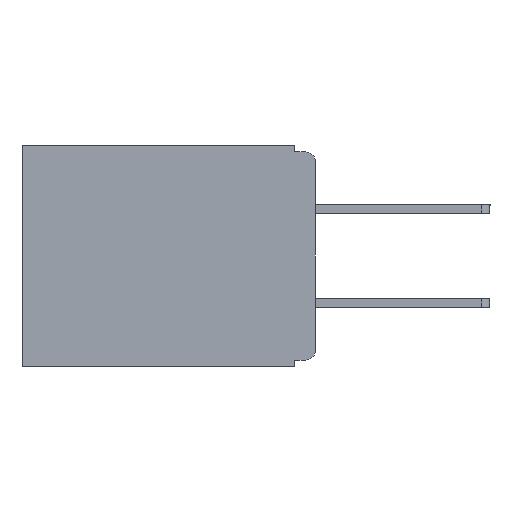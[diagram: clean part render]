
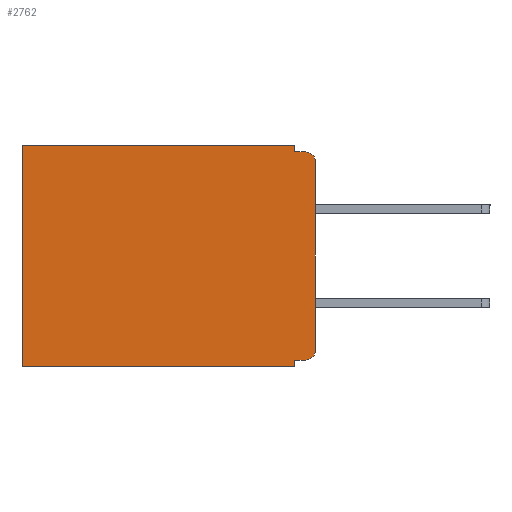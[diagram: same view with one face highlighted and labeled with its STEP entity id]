
A CAD part, left-side view. The second image highlights one B-rep face of the part: STEP entity #2762.
In plain terms, the highlighted planar face has unit normal (-1, 0, 0).
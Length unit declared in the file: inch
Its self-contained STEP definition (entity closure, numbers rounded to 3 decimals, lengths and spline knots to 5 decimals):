
#59 = CARTESIAN_POINT ( 'NONE',  ( 0.3, 0., -0.33 ) ) ;
#612 = CARTESIAN_POINT ( 'NONE',  ( 0.3, 0.015, -0.305 ) ) ;
#1297 = FACE_OUTER_BOUND ( 'NONE', #2068, .T. ) ;
#1448 = ORIENTED_EDGE ( 'NONE', *, *, #30061, .T. ) ;
#1868 = EDGE_CURVE ( 'NONE', #29486, #16507, #29975, .T. ) ;
#2068 = EDGE_LOOP ( 'NONE', ( #18898, #1448, #10422, #10959, #26774, #23212, #26796, #8528, #10632, #19428 ) ) ;
#2762 = ADVANCED_FACE ( 'NONE', ( #1297 ), #14230, .F. ) ;
#3107 = DIRECTION ( 'NONE',  ( 0., 0., -1. ) ) ;
#4763 = CARTESIAN_POINT ( 'NONE',  ( 0.3, 0., -0.305 ) ) ;
#4853 = EDGE_CURVE ( 'NONE', #28722, #25468, #7602, .T. ) ;
#6275 = VECTOR ( 'NONE', #17527, 39.37008 ) ;
#6367 = CARTESIAN_POINT ( 'NONE',  ( 0.3, 0., -0.32 ) ) ;
#6428 = CIRCLE ( 'NONE', #27168, 0.015 ) ;
#6595 = VERTEX_POINT ( 'NONE', #8997 ) ;
#6731 = DIRECTION ( 'NONE',  ( 0., 1., 0. ) ) ;
#6753 = CARTESIAN_POINT ( 'NONE',  ( 0.3, 0., -0.33 ) ) ;
#6764 = CARTESIAN_POINT ( 'NONE',  ( 0.3, 0.437, 0. ) ) ;
#6774 = LINE ( 'NONE', #8941, #23721 ) ;
#6775 = VECTOR ( 'NONE', #29089, 39.37008 ) ;
#6776 = LINE ( 'NONE', #6753, #12218 ) ;
#7475 = VERTEX_POINT ( 'NONE', #7831 ) ;
#7602 = LINE ( 'NONE', #6367, #13026 ) ;
#7777 = LINE ( 'NONE', #14402, #19295 ) ;
#7831 = CARTESIAN_POINT ( 'NONE',  ( 0.3, 0.031, -0.33 ) ) ;
#7839 = DIRECTION ( 'NONE',  ( 1., 0., 0. ) ) ;
#8376 = CARTESIAN_POINT ( 'NONE',  ( 0.3, 0., -0.01 ) ) ;
#8528 = ORIENTED_EDGE ( 'NONE', *, *, #25667, .F. ) ;
#8941 = CARTESIAN_POINT ( 'NONE',  ( 0.3, 0., 0. ) ) ;
#8997 = CARTESIAN_POINT ( 'NONE',  ( 0.3, 0.015, -0.01 ) ) ;
#9404 = AXIS2_PLACEMENT_3D ( 'NONE', #59, #7839, #13425 ) ;
#10422 = ORIENTED_EDGE ( 'NONE', *, *, #12628, .F. ) ;
#10632 = ORIENTED_EDGE ( 'NONE', *, *, #4853, .F. ) ;
#10792 = VERTEX_POINT ( 'NONE', #21966 ) ;
#10959 = ORIENTED_EDGE ( 'NONE', *, *, #27193, .F. ) ;
#11281 = DIRECTION ( 'NONE',  ( 0., 1., 0. ) ) ;
#11301 = VERTEX_POINT ( 'NONE', #16894 ) ;
#12197 = CIRCLE ( 'NONE', #25722, 0.015 ) ;
#12218 = VECTOR ( 'NONE', #18340, 39.37008 ) ;
#12562 = CARTESIAN_POINT ( 'NONE',  ( 0.3, 0.015, -0.025 ) ) ;
#12628 = EDGE_CURVE ( 'NONE', #19249, #6595, #17962, .T. ) ;
#12634 = CARTESIAN_POINT ( 'NONE',  ( 0.3, 0., -0.33 ) ) ;
#12815 = EDGE_CURVE ( 'NONE', #7475, #16507, #6776, .T. ) ;
#12888 = CARTESIAN_POINT ( 'NONE',  ( 0.3, 0.437, -0.33 ) ) ;
#13026 = VECTOR ( 'NONE', #6731, 39.37008 ) ;
#13425 = DIRECTION ( 'NONE',  ( 0., 0., -1. ) ) ;
#14230 = PLANE ( 'NONE',  #9404 ) ;
#14402 = CARTESIAN_POINT ( 'NONE',  ( 0.3, 0.031, 0. ) ) ;
#14833 = DIRECTION ( 'NONE',  ( 0., 0., -1. ) ) ;
#16507 = VERTEX_POINT ( 'NONE', #12888 ) ;
#16696 = DIRECTION ( 'NONE',  ( 0., 0., -1. ) ) ;
#16894 = CARTESIAN_POINT ( 'NONE',  ( 0.3, 0., -0.025 ) ) ;
#16998 = DIRECTION ( 'NONE',  ( -1., 0., 0. ) ) ;
#17232 = VECTOR ( 'NONE', #17438, 39.37008 ) ;
#17438 = DIRECTION ( 'NONE',  ( 0., -1., 0. ) ) ;
#17527 = DIRECTION ( 'NONE',  ( 0., 0., -1. ) ) ;
#17594 = CARTESIAN_POINT ( 'NONE',  ( 0.3, 0.031, -0.01 ) ) ;
#17962 = LINE ( 'NONE', #8376, #17232 ) ;
#18340 = DIRECTION ( 'NONE',  ( 0., 1., 0. ) ) ;
#18898 = ORIENTED_EDGE ( 'NONE', *, *, #20298, .F. ) ;
#19249 = VERTEX_POINT ( 'NONE', #17594 ) ;
#19295 = VECTOR ( 'NONE', #16696, 39.37008 ) ;
#19428 = ORIENTED_EDGE ( 'NONE', *, *, #25488, .T. ) ;
#19701 = CARTESIAN_POINT ( 'NONE',  ( 0.3, 0.437, -0.33 ) ) ;
#19743 = LINE ( 'NONE', #24447, #6775 ) ;
#19780 = CARTESIAN_POINT ( 'NONE',  ( 0.3, 0.015, -0.32 ) ) ;
#20298 = EDGE_CURVE ( 'NONE', #11301, #22526, #27330, .T. ) ;
#20519 = VECTOR ( 'NONE', #26351, 39.37008 ) ;
#21203 = EDGE_CURVE ( 'NONE', #10792, #29486, #6774, .T. ) ;
#21966 = CARTESIAN_POINT ( 'NONE',  ( 0.3, 0.031, 0. ) ) ;
#22526 = VERTEX_POINT ( 'NONE', #4763 ) ;
#23212 = ORIENTED_EDGE ( 'NONE', *, *, #1868, .T. ) ;
#23721 = VECTOR ( 'NONE', #11281, 39.37008 ) ;
#24447 = CARTESIAN_POINT ( 'NONE',  ( 0.3, 0.031, -0.33 ) ) ;
#25468 = VERTEX_POINT ( 'NONE', #28300 ) ;
#25488 = EDGE_CURVE ( 'NONE', #28722, #22526, #6428, .T. ) ;
#25667 = EDGE_CURVE ( 'NONE', #25468, #7475, #19743, .T. ) ;
#25722 = AXIS2_PLACEMENT_3D ( 'NONE', #12562, #28560, #14833 ) ;
#26351 = DIRECTION ( 'NONE',  ( 0., 0., -1. ) ) ;
#26774 = ORIENTED_EDGE ( 'NONE', *, *, #21203, .T. ) ;
#26796 = ORIENTED_EDGE ( 'NONE', *, *, #12815, .F. ) ;
#27168 = AXIS2_PLACEMENT_3D ( 'NONE', #612, #16998, #3107 ) ;
#27193 = EDGE_CURVE ( 'NONE', #10792, #19249, #7777, .T. ) ;
#27330 = LINE ( 'NONE', #12634, #20519 ) ;
#28300 = CARTESIAN_POINT ( 'NONE',  ( 0.3, 0.031, -0.32 ) ) ;
#28560 = DIRECTION ( 'NONE',  ( -1., 0., 0. ) ) ;
#28722 = VERTEX_POINT ( 'NONE', #19780 ) ;
#29089 = DIRECTION ( 'NONE',  ( 0., 0., -1. ) ) ;
#29486 = VERTEX_POINT ( 'NONE', #6764 ) ;
#29975 = LINE ( 'NONE', #19701, #6275 ) ;
#30061 = EDGE_CURVE ( 'NONE', #11301, #6595, #12197, .T. ) ;
